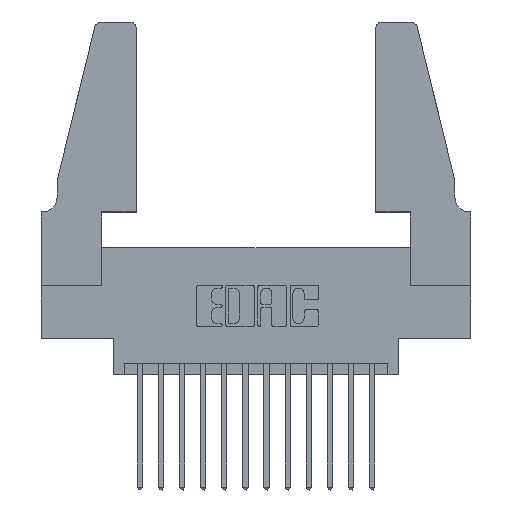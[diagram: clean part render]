
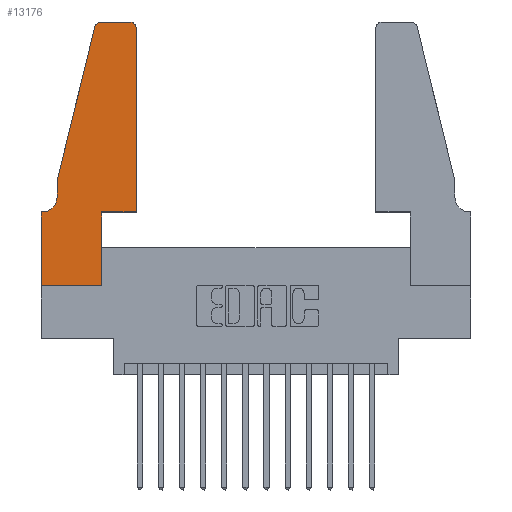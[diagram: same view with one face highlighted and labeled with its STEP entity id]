
A CAD part, top view. The second image highlights one B-rep face of the part: STEP entity #13176.
In plain terms, the highlighted planar face has unit normal (0, 0, 1).
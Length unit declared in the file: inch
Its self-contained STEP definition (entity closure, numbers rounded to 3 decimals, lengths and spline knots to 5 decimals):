
#155 = CIRCLE ( 'NONE', #1437, 0.03 ) ;
#342 = VECTOR ( 'NONE', #4682, 39.37008 ) ;
#373 = VECTOR ( 'NONE', #9400, 39.37008 ) ;
#492 = ORIENTED_EDGE ( 'NONE', *, *, #11112, .T. ) ;
#599 = VERTEX_POINT ( 'NONE', #12932 ) ;
#647 = AXIS2_PLACEMENT_3D ( 'NONE', #11557, #5461, #13930 ) ;
#972 = AXIS2_PLACEMENT_3D ( 'NONE', #7427, #15747, #8691 ) ;
#1240 = DIRECTION ( 'NONE',  ( 1., 0., 0. ) ) ;
#1266 = LINE ( 'NONE', #3187, #7945 ) ;
#1335 = CARTESIAN_POINT ( 'NONE',  ( 0.25487, 1.22718, 0.37 ) ) ;
#1381 = VECTOR ( 'NONE', #7640, 39.37008 ) ;
#1408 = ORIENTED_EDGE ( 'NONE', *, *, #3136, .T. ) ;
#1437 = AXIS2_PLACEMENT_3D ( 'NONE', #5499, #8754, #1240 ) ;
#1438 = VECTOR ( 'NONE', #6962, 39.37008 ) ;
#1649 = CARTESIAN_POINT ( 'NONE',  ( 0.0755, 0.5, 0.37 ) ) ;
#1704 = DIRECTION ( 'NONE',  ( 0., -1., 0. ) ) ;
#2707 = ORIENTED_EDGE ( 'NONE', *, *, #6725, .T. ) ;
#2782 = ORIENTED_EDGE ( 'NONE', *, *, #4904, .T. ) ;
#3075 = VERTEX_POINT ( 'NONE', #13397 ) ;
#3136 = EDGE_CURVE ( 'NONE', #10473, #7090, #8441, .T. ) ;
#3140 = CARTESIAN_POINT ( 'NONE',  ( 0.2865, 0.35, 0.37 ) ) ;
#3187 = CARTESIAN_POINT ( 'NONE',  ( 0.0755, 0.5, 0.37 ) ) ;
#3345 = VERTEX_POINT ( 'NONE', #9188 ) ;
#3420 = CARTESIAN_POINT ( 'NONE',  ( 0.4505, 0.35, 0.37 ) ) ;
#3677 = VERTEX_POINT ( 'NONE', #14960 ) ;
#3820 = EDGE_CURVE ( 'NONE', #3345, #3075, #8993, .T. ) ;
#3852 = VERTEX_POINT ( 'NONE', #13377 ) ;
#4137 = ORIENTED_EDGE ( 'NONE', *, *, #4972, .T. ) ;
#4286 = LINE ( 'NONE', #14778, #1381 ) ;
#4416 = DIRECTION ( 'NONE',  ( -0.239, -0.971, 0. ) ) ;
#4551 = DIRECTION ( 'NONE',  ( 1., 0., 0. ) ) ;
#4554 = CARTESIAN_POINT ( 'NONE',  ( 0.2865, 0.35, 0.37 ) ) ;
#4682 = DIRECTION ( 'NONE',  ( 0., 1., 0. ) ) ;
#4749 = LINE ( 'NONE', #14144, #1438 ) ;
#4794 = DIRECTION ( 'NONE',  ( 0., 0., -1. ) ) ;
#4904 = EDGE_CURVE ( 'NONE', #3852, #12643, #12664, .T. ) ;
#4972 = EDGE_CURVE ( 'NONE', #7090, #3345, #15396, .T. ) ;
#5212 = CARTESIAN_POINT ( 'NONE',  ( 0.284, 1.25, 0.37 ) ) ;
#5406 = VECTOR ( 'NONE', #14383, 39.37008 ) ;
#5449 = VECTOR ( 'NONE', #4551, 39.37008 ) ;
#5461 = DIRECTION ( 'NONE',  ( 0., 0., 1. ) ) ;
#5499 = CARTESIAN_POINT ( 'NONE',  ( 0.4205, 1.22, 0.37 ) ) ;
#5808 = VERTEX_POINT ( 'NONE', #10017 ) ;
#5990 = EDGE_LOOP ( 'NONE', ( #2707, #14384, #14202, #1408, #4137, #13891, #7328, #14811, #492, #7290, #2782, #9056 ) ) ;
#6178 = FACE_OUTER_BOUND ( 'NONE', #5990, .T. ) ;
#6361 = CIRCLE ( 'NONE', #972, 0.03 ) ;
#6655 = AXIS2_PLACEMENT_3D ( 'NONE', #12154, #4794, #13339 ) ;
#6725 = EDGE_CURVE ( 'NONE', #3677, #11519, #4749, .T. ) ;
#6962 = DIRECTION ( 'NONE',  ( -1., 0., 0. ) ) ;
#7090 = VERTEX_POINT ( 'NONE', #9053 ) ;
#7290 = ORIENTED_EDGE ( 'NONE', *, *, #12503, .T. ) ;
#7328 = ORIENTED_EDGE ( 'NONE', *, *, #8902, .T. ) ;
#7427 = CARTESIAN_POINT ( 'NONE',  ( 0.284, 1.22, 0.37 ) ) ;
#7640 = DIRECTION ( 'NONE',  ( 0., -1., 0. ) ) ;
#7945 = VECTOR ( 'NONE', #4416, 39.37008 ) ;
#8279 = CARTESIAN_POINT ( 'NONE',  ( 0., 0., 0.37 ) ) ;
#8441 = LINE ( 'NONE', #1649, #14363 ) ;
#8605 = VECTOR ( 'NONE', #14339, 39.37008 ) ;
#8691 = DIRECTION ( 'NONE',  ( 1., 0., 0. ) ) ;
#8754 = DIRECTION ( 'NONE',  ( 0., 0., 1. ) ) ;
#8902 = EDGE_CURVE ( 'NONE', #3075, #5808, #4286, .T. ) ;
#8993 = LINE ( 'NONE', #14840, #8605 ) ;
#9053 = CARTESIAN_POINT ( 'NONE',  ( 0.0755, 0.42, 0.37 ) ) ;
#9056 = ORIENTED_EDGE ( 'NONE', *, *, #10760, .T. ) ;
#9188 = CARTESIAN_POINT ( 'NONE',  ( 0.0055, 0.35, 0.37 ) ) ;
#9400 = DIRECTION ( 'NONE',  ( 0., 1., 0. ) ) ;
#10006 = VERTEX_POINT ( 'NONE', #4554 ) ;
#10017 = CARTESIAN_POINT ( 'NONE',  ( 0., 0., 0.37 ) ) ;
#10373 = PLANE ( 'NONE',  #647 ) ;
#10473 = VERTEX_POINT ( 'NONE', #10596 ) ;
#10581 = EDGE_CURVE ( 'NONE', #5808, #599, #15064, .T. ) ;
#10596 = CARTESIAN_POINT ( 'NONE',  ( 0.0755, 0.5, 0.37 ) ) ;
#10760 = EDGE_CURVE ( 'NONE', #12643, #3677, #155, .T. ) ;
#11112 = EDGE_CURVE ( 'NONE', #599, #10006, #13795, .T. ) ;
#11519 = VERTEX_POINT ( 'NONE', #5212 ) ;
#11557 = CARTESIAN_POINT ( 'NONE',  ( 0., 0.35, 0.37 ) ) ;
#12045 = CARTESIAN_POINT ( 'NONE',  ( 0.4505, 0.35, 0.37 ) ) ;
#12154 = CARTESIAN_POINT ( 'NONE',  ( 0.0055, 0.42, 0.37 ) ) ;
#12503 = EDGE_CURVE ( 'NONE', #10006, #3852, #15023, .T. ) ;
#12643 = VERTEX_POINT ( 'NONE', #13418 ) ;
#12664 = LINE ( 'NONE', #12045, #342 ) ;
#12703 = VERTEX_POINT ( 'NONE', #1335 ) ;
#12932 = CARTESIAN_POINT ( 'NONE',  ( 0.2865, 0., 0.37 ) ) ;
#12997 = EDGE_CURVE ( 'NONE', #12703, #10473, #1266, .T. ) ;
#13176 = ADVANCED_FACE ( 'NONE', ( #6178 ), #10373, .T. ) ;
#13339 = DIRECTION ( 'NONE',  ( -1., 0., 0. ) ) ;
#13377 = CARTESIAN_POINT ( 'NONE',  ( 0.4505, 0.35, 0.37 ) ) ;
#13397 = CARTESIAN_POINT ( 'NONE',  ( 0., 0.35, 0.37 ) ) ;
#13418 = CARTESIAN_POINT ( 'NONE',  ( 0.4505, 1.22, 0.37 ) ) ;
#13795 = LINE ( 'NONE', #3140, #373 ) ;
#13891 = ORIENTED_EDGE ( 'NONE', *, *, #3820, .T. ) ;
#13930 = DIRECTION ( 'NONE',  ( 1., 0., 0. ) ) ;
#14144 = CARTESIAN_POINT ( 'NONE',  ( 0.2605, 1.25, 0.37 ) ) ;
#14202 = ORIENTED_EDGE ( 'NONE', *, *, #12997, .T. ) ;
#14339 = DIRECTION ( 'NONE',  ( -1., 0., 0. ) ) ;
#14363 = VECTOR ( 'NONE', #1704, 39.37008 ) ;
#14383 = DIRECTION ( 'NONE',  ( 1., 0., 0. ) ) ;
#14384 = ORIENTED_EDGE ( 'NONE', *, *, #15289, .T. ) ;
#14778 = CARTESIAN_POINT ( 'NONE',  ( 0., 0., 0.37 ) ) ;
#14811 = ORIENTED_EDGE ( 'NONE', *, *, #10581, .T. ) ;
#14840 = CARTESIAN_POINT ( 'NONE',  ( 0.0755, 0.35, 0.37 ) ) ;
#14960 = CARTESIAN_POINT ( 'NONE',  ( 0.4205, 1.25, 0.37 ) ) ;
#15023 = LINE ( 'NONE', #3420, #5406 ) ;
#15064 = LINE ( 'NONE', #8279, #5449 ) ;
#15289 = EDGE_CURVE ( 'NONE', #11519, #12703, #6361, .T. ) ;
#15396 = CIRCLE ( 'NONE', #6655, 0.07 ) ;
#15747 = DIRECTION ( 'NONE',  ( 0., 0., 1. ) ) ;
